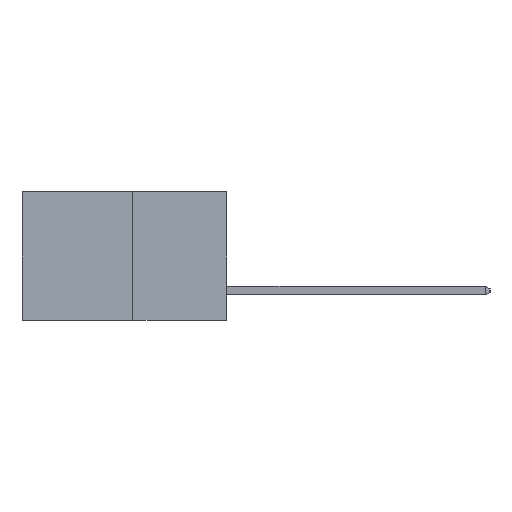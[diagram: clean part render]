
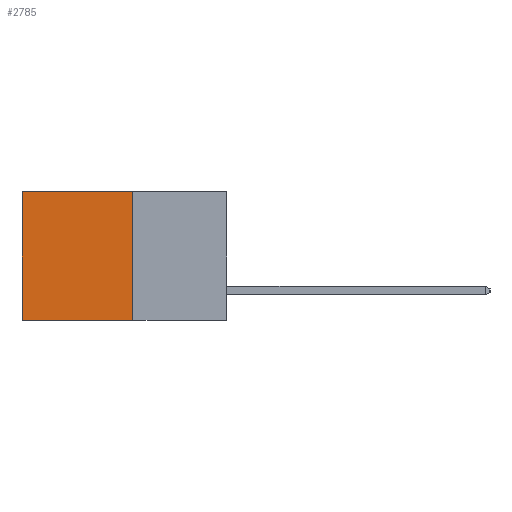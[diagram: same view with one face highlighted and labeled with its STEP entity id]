
A CAD part, left-side view. The second image highlights one B-rep face of the part: STEP entity #2785.
In plain terms, the highlighted planar face has unit normal (-1, 0, 0).
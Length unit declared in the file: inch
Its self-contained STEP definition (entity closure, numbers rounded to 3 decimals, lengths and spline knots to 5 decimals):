
#502 = EDGE_CURVE ( 'NONE', #4407, #5931, #5679, .T. ) ;
#615 = CARTESIAN_POINT ( 'NONE',  ( 0.277, 0.27, -0.37 ) ) ;
#772 = FACE_OUTER_BOUND ( 'NONE', #2103, .T. ) ;
#899 = LINE ( 'NONE', #615, #7087 ) ;
#1457 = EDGE_CURVE ( 'NONE', #2937, #4407, #899, .T. ) ;
#1482 = EDGE_CURVE ( 'NONE', #2937, #2184, #2479, .T. ) ;
#1616 = DIRECTION ( 'NONE',  ( 0., 0., -1. ) ) ;
#2027 = DIRECTION ( 'NONE',  ( 1., 0., 0. ) ) ;
#2028 = DIRECTION ( 'NONE',  ( 0., 0., -1. ) ) ;
#2089 = PLANE ( 'NONE',  #8710 ) ;
#2103 = EDGE_LOOP ( 'NONE', ( #6131, #6073, #6050, #5992 ) ) ;
#2133 = CARTESIAN_POINT ( 'NONE',  ( 0.277, 0.27, -0.37 ) ) ;
#2184 = VERTEX_POINT ( 'NONE', #8325 ) ;
#2479 = LINE ( 'NONE', #7722, #4365 ) ;
#2785 = ADVANCED_FACE ( 'NONE', ( #772 ), #2089, .F. ) ;
#2937 = VERTEX_POINT ( 'NONE', #7157 ) ;
#2953 = CARTESIAN_POINT ( 'NONE',  ( 0.277, 0.27, -0.37 ) ) ;
#3476 = DIRECTION ( 'NONE',  ( 0., 1., 0. ) ) ;
#4365 = VECTOR ( 'NONE', #3476, 39.37008 ) ;
#4407 = VERTEX_POINT ( 'NONE', #2953 ) ;
#4467 = CARTESIAN_POINT ( 'NONE',  ( 0.277, 0.59, -0.37 ) ) ;
#4982 = EDGE_CURVE ( 'NONE', #2184, #5931, #5973, .T. ) ;
#5045 = CARTESIAN_POINT ( 'NONE',  ( 0.277, 0.59, -0.37 ) ) ;
#5392 = DIRECTION ( 'NONE',  ( 0., 0., -1. ) ) ;
#5678 = CARTESIAN_POINT ( 'NONE',  ( 0.277, 0.27, -0.37 ) ) ;
#5679 = LINE ( 'NONE', #5678, #8951 ) ;
#5931 = VERTEX_POINT ( 'NONE', #4467 ) ;
#5973 = LINE ( 'NONE', #5045, #7762 ) ;
#5992 = ORIENTED_EDGE ( 'NONE', *, *, #1482, .T. ) ;
#6050 = ORIENTED_EDGE ( 'NONE', *, *, #1457, .F. ) ;
#6073 = ORIENTED_EDGE ( 'NONE', *, *, #502, .F. ) ;
#6131 = ORIENTED_EDGE ( 'NONE', *, *, #4982, .T. ) ;
#7087 = VECTOR ( 'NONE', #1616, 39.37008 ) ;
#7157 = CARTESIAN_POINT ( 'NONE',  ( 0.277, 0.27, 0. ) ) ;
#7722 = CARTESIAN_POINT ( 'NONE',  ( 0.277, 0.27, 0. ) ) ;
#7740 = DIRECTION ( 'NONE',  ( 0., 1., 0. ) ) ;
#7762 = VECTOR ( 'NONE', #5392, 39.37008 ) ;
#8325 = CARTESIAN_POINT ( 'NONE',  ( 0.277, 0.59, 0. ) ) ;
#8710 = AXIS2_PLACEMENT_3D ( 'NONE', #2133, #2027, #2028 ) ;
#8951 = VECTOR ( 'NONE', #7740, 39.37008 ) ;
